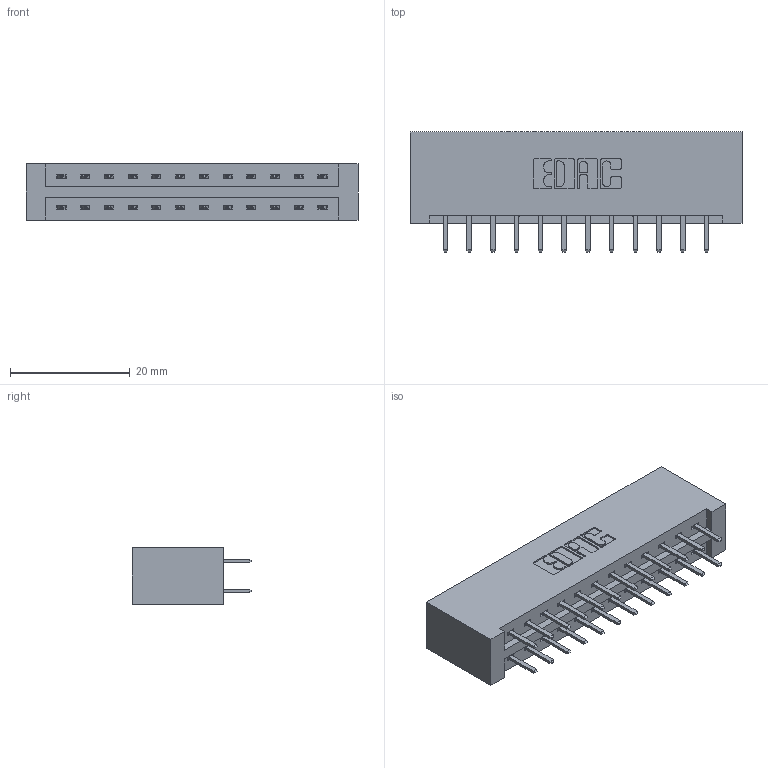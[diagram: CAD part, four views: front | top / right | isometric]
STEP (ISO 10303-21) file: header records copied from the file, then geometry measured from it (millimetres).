
FILE_DESCRIPTION (( 'STEP AP203' ), '1' );
FILE_NAME ('337-024-520-201.STEP', '2018-08-05T18:17:12', ( '' ), ( '' ), 'SwSTEP 2.0', 'SolidWorks 2016', '' );
FILE_SCHEMA (( 'CONFIG_CONTROL_DESIGN' ));
Length unit declared in the file: inch
Products named in the file (3): 337 Part_No Mounting Lugs; 345-292-001_345-293-120; 337-024-520-201
Assembly tree (25 placements, depth 2):
  337-024-520-201
    337 Part_No Mounting Lugs
    345-292-001_345-293-120  x24
Bounding box: 55.42 x 20.02 x 9.4 mm (x, y, z)
Volume: 6191.8 mm3; surface area: 6734.4 mm2
Topology: 25 solids, 25 shells, 1498 faces, 4343 edges, 2830 vertices
Faces by surface type: plane 1026, cylinder 472
Entity records: 13021 total; most frequent: CARTESIAN_POINT 2230, ORIENTED_EDGE 2154, DIRECTION 1933, EDGE_CURVE 1077, VECTOR 953, LINE 953, VERTEX_POINT 714, AXIS2_PLACEMENT_3D 490
